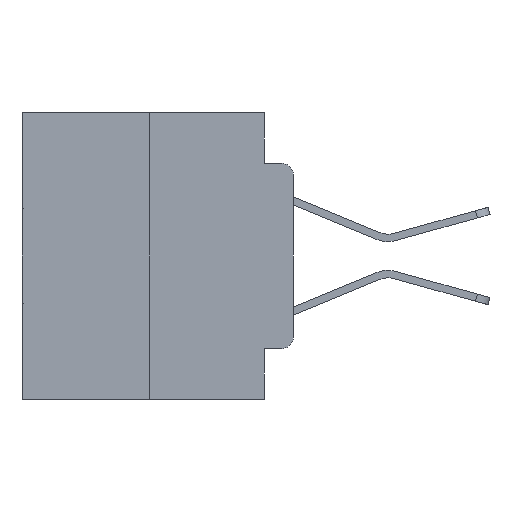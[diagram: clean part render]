
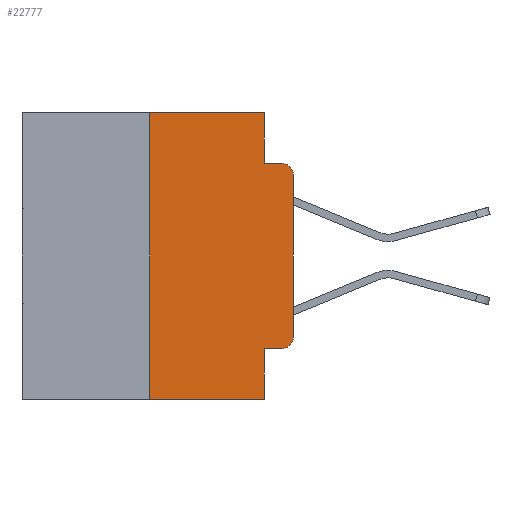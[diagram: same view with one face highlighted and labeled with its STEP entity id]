
A CAD part, left-side view. The second image highlights one B-rep face of the part: STEP entity #22777.
In plain terms, the highlighted planar face has unit normal (-1, 0, 0).
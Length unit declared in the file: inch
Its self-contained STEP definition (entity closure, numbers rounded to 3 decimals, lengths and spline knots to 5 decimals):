
#986 = ORIENTED_EDGE ( 'NONE', *, *, #9680, .F. ) ;
#1324 = LINE ( 'NONE', #16618, #5062 ) ;
#1486 = VERTEX_POINT ( 'NONE', #8768 ) ;
#1614 = ORIENTED_EDGE ( 'NONE', *, *, #18599, .F. ) ;
#2074 = LINE ( 'NONE', #17814, #10415 ) ;
#2691 = CARTESIAN_POINT ( 'NONE',  ( 0., 0.473, 0. ) ) ;
#3489 = LINE ( 'NONE', #12442, #6439 ) ;
#3553 = CARTESIAN_POINT ( 'NONE',  ( 0., 0.02, -0.1085 ) ) ;
#3619 = PLANE ( 'NONE',  #27604 ) ;
#3932 = CARTESIAN_POINT ( 'NONE',  ( 0., 0.02, -0.3915 ) ) ;
#4084 = DIRECTION ( 'NONE',  ( -1., 0., 0. ) ) ;
#4211 = ORIENTED_EDGE ( 'NONE', *, *, #8204, .T. ) ;
#5062 = VECTOR ( 'NONE', #15006, 39.37008 ) ;
#5360 = LINE ( 'NONE', #14344, #8240 ) ;
#5525 = CARTESIAN_POINT ( 'NONE',  ( 0., 0.473, 0. ) ) ;
#5780 = CARTESIAN_POINT ( 'NONE',  ( 0., 0.051, -0.0885 ) ) ;
#6107 = DIRECTION ( 'NONE',  ( 1., 0., 0. ) ) ;
#6439 = VECTOR ( 'NONE', #16436, 39.37008 ) ;
#6727 = VECTOR ( 'NONE', #17517, 39.37008 ) ;
#7294 = CIRCLE ( 'NONE', #22299, 0.02 ) ;
#7456 = DIRECTION ( 'NONE',  ( 0., 0., -1. ) ) ;
#7834 = EDGE_CURVE ( 'NONE', #1486, #28110, #19311, .T. ) ;
#8204 = EDGE_CURVE ( 'NONE', #23628, #28110, #7294, .T. ) ;
#8240 = VECTOR ( 'NONE', #14198, 39.37008 ) ;
#8257 = AXIS2_PLACEMENT_3D ( 'NONE', #3932, #4084, #13052 ) ;
#8314 = DIRECTION ( 'NONE',  ( 0., 0., -1. ) ) ;
#8768 = CARTESIAN_POINT ( 'NONE',  ( 0., 0.051, -0.0885 ) ) ;
#9680 = EDGE_CURVE ( 'NONE', #21870, #1486, #3489, .T. ) ;
#10415 = VECTOR ( 'NONE', #7456, 39.37008 ) ;
#10641 = VERTEX_POINT ( 'NONE', #16757 ) ;
#12229 = EDGE_CURVE ( 'NONE', #26062, #16868, #2074, .T. ) ;
#12308 = CARTESIAN_POINT ( 'NONE',  ( 0., 0.02, -0.0885 ) ) ;
#12442 = CARTESIAN_POINT ( 'NONE',  ( 0., 0.051, 0. ) ) ;
#13052 = DIRECTION ( 'NONE',  ( 0., 0., -1. ) ) ;
#13179 = CARTESIAN_POINT ( 'NONE',  ( 0., 0.051, -0.4115 ) ) ;
#14198 = DIRECTION ( 'NONE',  ( 0., 0., 1. ) ) ;
#14344 = CARTESIAN_POINT ( 'NONE',  ( 0., 0.25, 0. ) ) ;
#14517 = ORIENTED_EDGE ( 'NONE', *, *, #25141, .T. ) ;
#14530 = ORIENTED_EDGE ( 'NONE', *, *, #25862, .T. ) ;
#14747 = CARTESIAN_POINT ( 'NONE',  ( 0., 0.25, -0.5 ) ) ;
#14785 = VECTOR ( 'NONE', #18111, 39.37008 ) ;
#15006 = DIRECTION ( 'NONE',  ( 0., -1., 0. ) ) ;
#15816 = ORIENTED_EDGE ( 'NONE', *, *, #12229, .F. ) ;
#16058 = LINE ( 'NONE', #2691, #14785 ) ;
#16179 = VECTOR ( 'NONE', #16858, 39.37008 ) ;
#16436 = DIRECTION ( 'NONE',  ( 0., 0., -1. ) ) ;
#16618 = CARTESIAN_POINT ( 'NONE',  ( 0., 0.473, -0.5 ) ) ;
#16757 = CARTESIAN_POINT ( 'NONE',  ( 0., 0., -0.3915 ) ) ;
#16858 = DIRECTION ( 'NONE',  ( 0., 0., 1. ) ) ;
#16868 = VERTEX_POINT ( 'NONE', #22127 ) ;
#16928 = DIRECTION ( 'NONE',  ( 0., 0., -1. ) ) ;
#17366 = CARTESIAN_POINT ( 'NONE',  ( 0., 0.25, 0. ) ) ;
#17517 = DIRECTION ( 'NONE',  ( 0., -1., 0. ) ) ;
#17519 = ORIENTED_EDGE ( 'NONE', *, *, #7834, .F. ) ;
#17814 = CARTESIAN_POINT ( 'NONE',  ( 0., 0.051, 0. ) ) ;
#18111 = DIRECTION ( 'NONE',  ( 0., -1., 0. ) ) ;
#18268 = CARTESIAN_POINT ( 'NONE',  ( 0., 0.02, -0.4115 ) ) ;
#18599 = EDGE_CURVE ( 'NONE', #23801, #21870, #16058, .T. ) ;
#19060 = CARTESIAN_POINT ( 'NONE',  ( 0., 0., 0. ) ) ;
#19311 = LINE ( 'NONE', #5780, #25360 ) ;
#19402 = ORIENTED_EDGE ( 'NONE', *, *, #21788, .T. ) ;
#19450 = EDGE_CURVE ( 'NONE', #21335, #23801, #5360, .T. ) ;
#19846 = CARTESIAN_POINT ( 'NONE',  ( 0., 0.051, -0.4115 ) ) ;
#20718 = ORIENTED_EDGE ( 'NONE', *, *, #19450, .F. ) ;
#21335 = VERTEX_POINT ( 'NONE', #14747 ) ;
#21788 = EDGE_CURVE ( 'NONE', #21335, #16868, #1324, .T. ) ;
#21870 = VERTEX_POINT ( 'NONE', #28635 ) ;
#22127 = CARTESIAN_POINT ( 'NONE',  ( 0., 0.051, -0.5 ) ) ;
#22299 = AXIS2_PLACEMENT_3D ( 'NONE', #3553, #28079, #16928 ) ;
#22777 = ADVANCED_FACE ( 'NONE', ( #28420 ), #3619, .F. ) ;
#23014 = LINE ( 'NONE', #19060, #16179 ) ;
#23628 = VERTEX_POINT ( 'NONE', #27483 ) ;
#23688 = DIRECTION ( 'NONE',  ( 0., -1., 0. ) ) ;
#23801 = VERTEX_POINT ( 'NONE', #17366 ) ;
#24290 = EDGE_LOOP ( 'NONE', ( #14530, #4211, #17519, #986, #1614, #20718, #19402, #15816, #14517, #26306 ) ) ;
#25141 = EDGE_CURVE ( 'NONE', #26062, #27583, #28651, .T. ) ;
#25360 = VECTOR ( 'NONE', #23688, 39.37008 ) ;
#25585 = CIRCLE ( 'NONE', #8257, 0.02 ) ;
#25862 = EDGE_CURVE ( 'NONE', #10641, #23628, #23014, .T. ) ;
#26062 = VERTEX_POINT ( 'NONE', #13179 ) ;
#26306 = ORIENTED_EDGE ( 'NONE', *, *, #27097, .T. ) ;
#27097 = EDGE_CURVE ( 'NONE', #27583, #10641, #25585, .T. ) ;
#27483 = CARTESIAN_POINT ( 'NONE',  ( 0., 0., -0.1085 ) ) ;
#27583 = VERTEX_POINT ( 'NONE', #18268 ) ;
#27604 = AXIS2_PLACEMENT_3D ( 'NONE', #5525, #6107, #8314 ) ;
#28079 = DIRECTION ( 'NONE',  ( -1., 0., 0. ) ) ;
#28110 = VERTEX_POINT ( 'NONE', #12308 ) ;
#28420 = FACE_OUTER_BOUND ( 'NONE', #24290, .T. ) ;
#28635 = CARTESIAN_POINT ( 'NONE',  ( 0., 0.051, 0. ) ) ;
#28651 = LINE ( 'NONE', #19846, #6727 ) ;
